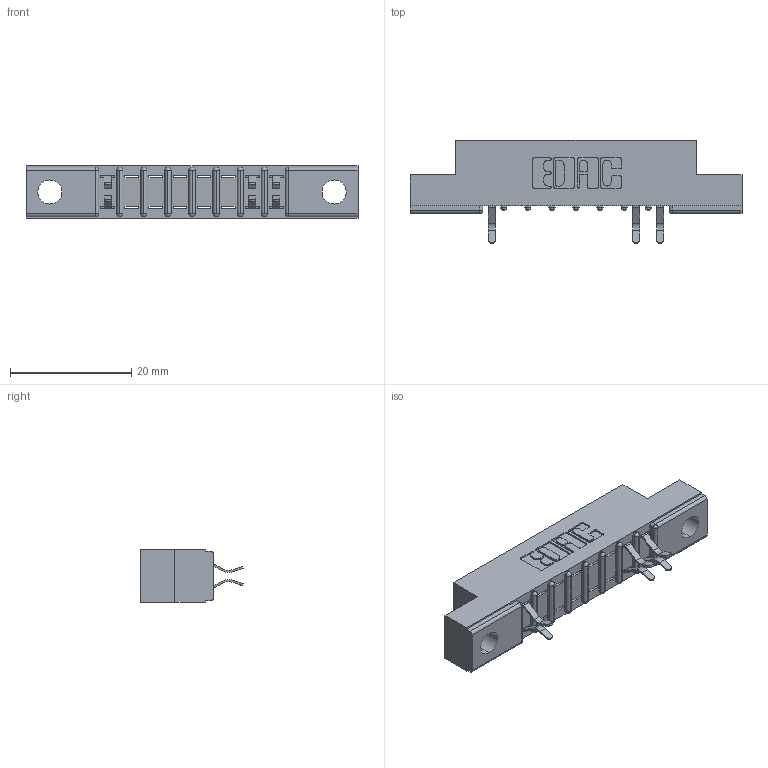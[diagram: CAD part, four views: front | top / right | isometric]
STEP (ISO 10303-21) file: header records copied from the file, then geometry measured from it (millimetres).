
FILE_DESCRIPTION (( 'STEP AP203' ), '1' );
FILE_NAME ('357-016-556-204.STEP', '2018-08-08T03:01:14', ( '' ), ( '' ), 'SwSTEP 2.0', 'SolidWorks 2016', '' );
FILE_SCHEMA (( 'CONFIG_CONTROL_DESIGN' ));
Length unit declared in the file: inch
Products named in the file (3): 307 Part_.156 Dia Mounting Holes; 307-290-001_556; 357-016-556-204
Assembly tree (7 placements, depth 2):
  357-016-556-204
    307 Part_.156 Dia Mounting Holes
    307-290-001_556  x6
Bounding box: 54.71 x 16.97 x 8.71 mm (x, y, z)
Volume: 3343.8 mm3; surface area: 4293.7 mm2
Topology: 7 solids, 7 shells, 541 faces, 1531 edges, 986 vertices
Faces by surface type: plane 342, cylinder 181, sphere 18
Entity records: 11508 total; most frequent: CARTESIAN_POINT 1940, ORIENTED_EDGE 1926, DIRECTION 1897, EDGE_CURVE 963, VECTOR 731, LINE 731, VERTEX_POINT 626, AXIS2_PLACEMENT_3D 583
